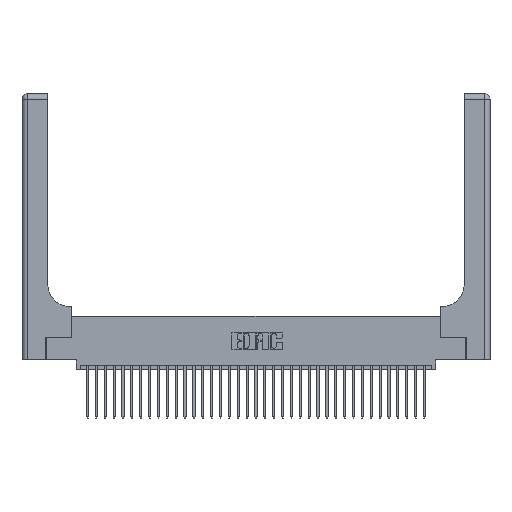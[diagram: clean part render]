
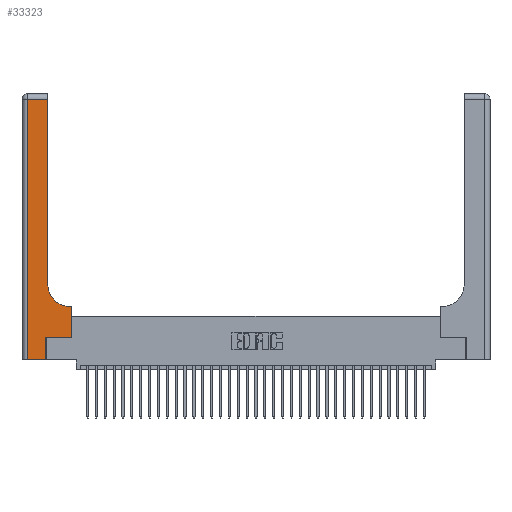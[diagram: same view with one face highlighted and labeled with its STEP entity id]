
A CAD part, top view. The second image highlights one B-rep face of the part: STEP entity #33323.
In plain terms, the highlighted planar face has unit normal (0, 0, 1).
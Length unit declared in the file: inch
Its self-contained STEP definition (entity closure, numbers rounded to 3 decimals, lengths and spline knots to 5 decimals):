
#159 = VECTOR ( 'NONE', #31679, 39.37008 ) ;
#726 = VERTEX_POINT ( 'NONE', #34015 ) ;
#1011 = AXIS2_PLACEMENT_3D ( 'NONE', #29072, #1086, #20865 ) ;
#1086 = DIRECTION ( 'NONE',  ( 0., 0., -1. ) ) ;
#1741 = EDGE_CURVE ( 'NONE', #27174, #7846, #33554, .T. ) ;
#2039 = ORIENTED_EDGE ( 'NONE', *, *, #14461, .T. ) ;
#2294 = EDGE_CURVE ( 'NONE', #726, #13765, #19577, .T. ) ;
#2821 = VERTEX_POINT ( 'NONE', #4291 ) ;
#2950 = CARTESIAN_POINT ( 'NONE',  ( 0.5585, 0.25, 0.37 ) ) ;
#3050 = DIRECTION ( 'NONE',  ( 0., -1., 0. ) ) ;
#3831 = CARTESIAN_POINT ( 'NONE',  ( 0.5585, 0.6, 0.37 ) ) ;
#4291 = CARTESIAN_POINT ( 'NONE',  ( 0.2915, 0.85, 0.37 ) ) ;
#4643 = LINE ( 'NONE', #13576, #25462 ) ;
#6777 = EDGE_CURVE ( 'NONE', #13765, #20741, #4643, .T. ) ;
#6878 = ORIENTED_EDGE ( 'NONE', *, *, #1741, .T. ) ;
#7846 = VERTEX_POINT ( 'NONE', #3831 ) ;
#9390 = EDGE_CURVE ( 'NONE', #14731, #2821, #13369, .T. ) ;
#9852 = EDGE_CURVE ( 'NONE', #24970, #726, #18204, .T. ) ;
#10582 = CARTESIAN_POINT ( 'NONE',  ( 0.2915, 0.6, 0.37 ) ) ;
#10910 = CARTESIAN_POINT ( 'NONE',  ( 0.269, 0.25, 0.37 ) ) ;
#13369 = CIRCLE ( 'NONE', #22750, 0.25 ) ;
#13576 = CARTESIAN_POINT ( 'NONE',  ( 0., 0., 0.37 ) ) ;
#13698 = CARTESIAN_POINT ( 'NONE',  ( 0.5415, 0.6, 0.37 ) ) ;
#13765 = VERTEX_POINT ( 'NONE', #35743 ) ;
#13961 = ORIENTED_EDGE ( 'NONE', *, *, #31673, .T. ) ;
#14391 = CARTESIAN_POINT ( 'NONE',  ( 0.5415, 0.85, 0.37 ) ) ;
#14461 = EDGE_CURVE ( 'NONE', #7846, #14731, #34961, .T. ) ;
#14731 = VERTEX_POINT ( 'NONE', #13698 ) ;
#14903 = DIRECTION ( 'NONE',  ( 0., 1., 0. ) ) ;
#15172 = VECTOR ( 'NONE', #14903, 39.37008 ) ;
#16856 = ORIENTED_EDGE ( 'NONE', *, *, #2294, .T. ) ;
#17238 = DIRECTION ( 'NONE',  ( 1., 0., 0. ) ) ;
#18204 = LINE ( 'NONE', #22044, #32219 ) ;
#18668 = VECTOR ( 'NONE', #28500, 39.37008 ) ;
#18730 = CARTESIAN_POINT ( 'NONE',  ( 0.2915, 3., 0.37 ) ) ;
#19577 = LINE ( 'NONE', #25686, #33556 ) ;
#19646 = EDGE_CURVE ( 'NONE', #20741, #28406, #30119, .T. ) ;
#19719 = CARTESIAN_POINT ( 'NONE',  ( 0.269, 0., 0.37 ) ) ;
#19997 = EDGE_LOOP ( 'NONE', ( #21523, #29624, #16856, #22136, #25466, #13961, #6878, #2039, #23838 ) ) ;
#20376 = FACE_OUTER_BOUND ( 'NONE', #19997, .T. ) ;
#20741 = VERTEX_POINT ( 'NONE', #19719 ) ;
#20865 = DIRECTION ( 'NONE',  ( -1., 0., 0. ) ) ;
#21523 = ORIENTED_EDGE ( 'NONE', *, *, #35526, .T. ) ;
#21600 = DIRECTION ( 'NONE',  ( 0., 1., 0. ) ) ;
#22044 = CARTESIAN_POINT ( 'NONE',  ( 0., 2.94, 0.37 ) ) ;
#22136 = ORIENTED_EDGE ( 'NONE', *, *, #6777, .T. ) ;
#22750 = AXIS2_PLACEMENT_3D ( 'NONE', #14391, #33977, #17238 ) ;
#22926 = VECTOR ( 'NONE', #21600, 39.37008 ) ;
#23633 = LINE ( 'NONE', #28896, #159 ) ;
#23838 = ORIENTED_EDGE ( 'NONE', *, *, #9390, .T. ) ;
#24970 = VERTEX_POINT ( 'NONE', #31480 ) ;
#24981 = DIRECTION ( 'NONE',  ( 1., 0., 0. ) ) ;
#25462 = VECTOR ( 'NONE', #24981, 39.37008 ) ;
#25466 = ORIENTED_EDGE ( 'NONE', *, *, #19646, .T. ) ;
#25686 = CARTESIAN_POINT ( 'NONE',  ( 0.06, 3., 0.37 ) ) ;
#25732 = CARTESIAN_POINT ( 'NONE',  ( 0.5585, 0.25, 0.37 ) ) ;
#27174 = VERTEX_POINT ( 'NONE', #2950 ) ;
#27550 = DIRECTION ( 'NONE',  ( -1., 0., 0. ) ) ;
#27618 = VECTOR ( 'NONE', #33046, 39.37008 ) ;
#28406 = VERTEX_POINT ( 'NONE', #10910 ) ;
#28500 = DIRECTION ( 'NONE',  ( 0., 1., 0. ) ) ;
#28896 = CARTESIAN_POINT ( 'NONE',  ( 0.269, 0.25, 0.37 ) ) ;
#29072 = CARTESIAN_POINT ( 'NONE',  ( 0., 3., 0.37 ) ) ;
#29624 = ORIENTED_EDGE ( 'NONE', *, *, #9852, .T. ) ;
#30119 = LINE ( 'NONE', #34489, #15172 ) ;
#31480 = CARTESIAN_POINT ( 'NONE',  ( 0.2915, 2.94, 0.37 ) ) ;
#31673 = EDGE_CURVE ( 'NONE', #28406, #27174, #23633, .T. ) ;
#31679 = DIRECTION ( 'NONE',  ( 1., 0., 0. ) ) ;
#32219 = VECTOR ( 'NONE', #27550, 39.37008 ) ;
#33046 = DIRECTION ( 'NONE',  ( -1., 0., 0. ) ) ;
#33323 = ADVANCED_FACE ( 'NONE', ( #20376 ), #34756, .F. ) ;
#33554 = LINE ( 'NONE', #25732, #18668 ) ;
#33556 = VECTOR ( 'NONE', #3050, 39.37008 ) ;
#33977 = DIRECTION ( 'NONE',  ( 0., 0., -1. ) ) ;
#34015 = CARTESIAN_POINT ( 'NONE',  ( 0.06, 2.94, 0.37 ) ) ;
#34489 = CARTESIAN_POINT ( 'NONE',  ( 0.269, 0., 0.37 ) ) ;
#34756 = PLANE ( 'NONE',  #1011 ) ;
#34961 = LINE ( 'NONE', #10582, #27618 ) ;
#35055 = LINE ( 'NONE', #18730, #22926 ) ;
#35526 = EDGE_CURVE ( 'NONE', #2821, #24970, #35055, .T. ) ;
#35743 = CARTESIAN_POINT ( 'NONE',  ( 0.06, 0., 0.37 ) ) ;
